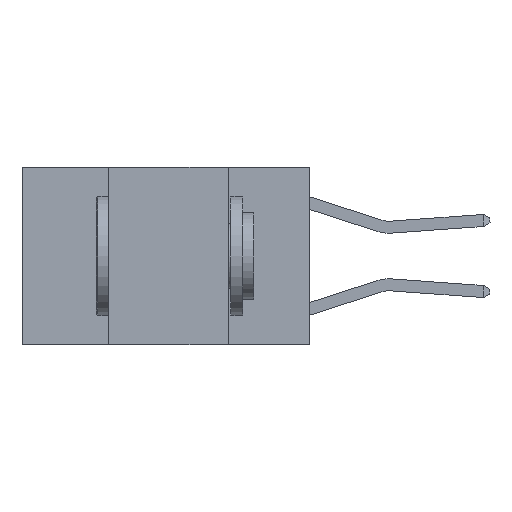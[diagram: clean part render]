
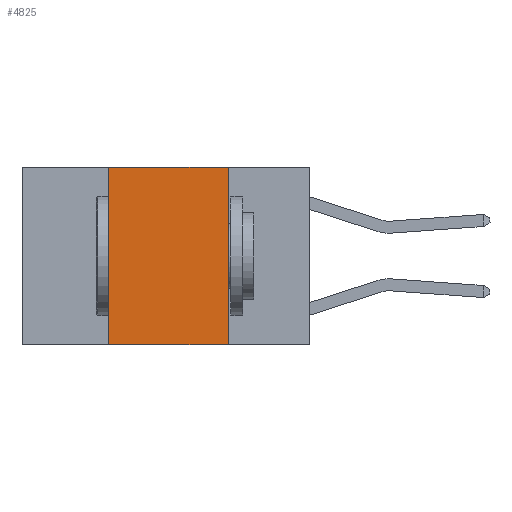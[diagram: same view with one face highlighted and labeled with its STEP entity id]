
A CAD part, left-side view. The second image highlights one B-rep face of the part: STEP entity #4825.
In plain terms, the highlighted planar face has unit normal (-1, 0, 0).
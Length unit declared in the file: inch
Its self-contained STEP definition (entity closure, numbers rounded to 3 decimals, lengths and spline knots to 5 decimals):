
#634 = VECTOR ( 'NONE', #3874, 39.37008 ) ;
#703 = VERTEX_POINT ( 'NONE', #14849 ) ;
#2016 = AXIS2_PLACEMENT_3D ( 'NONE', #13843, #4332, #15391 ) ;
#2614 = DIRECTION ( 'NONE',  ( 0., 0., 1. ) ) ;
#3172 = CARTESIAN_POINT ( 'NONE',  ( 0., 0.42, 0. ) ) ;
#3627 = CARTESIAN_POINT ( 'NONE',  ( 0., 0.6, -0.37 ) ) ;
#3639 = VECTOR ( 'NONE', #2614, 39.37008 ) ;
#3651 = ORIENTED_EDGE ( 'NONE', *, *, #3900, .F. ) ;
#3874 = DIRECTION ( 'NONE',  ( 0., 0., -1. ) ) ;
#3900 = EDGE_CURVE ( 'NONE', #703, #5578, #4510, .T. ) ;
#3946 = ORIENTED_EDGE ( 'NONE', *, *, #17797, .F. ) ;
#4332 = DIRECTION ( 'NONE',  ( 1., 0., 0. ) ) ;
#4471 = ORIENTED_EDGE ( 'NONE', *, *, #7173, .F. ) ;
#4510 = LINE ( 'NONE', #13406, #634 ) ;
#4579 = ORIENTED_EDGE ( 'NONE', *, *, #13881, .T. ) ;
#4668 = CARTESIAN_POINT ( 'NONE',  ( 0., 0.17, -0.37 ) ) ;
#4825 = ADVANCED_FACE ( 'NONE', ( #5985 ), #18412, .F. ) ;
#5578 = VERTEX_POINT ( 'NONE', #4668 ) ;
#5985 = FACE_OUTER_BOUND ( 'NONE', #7747, .T. ) ;
#7173 = EDGE_CURVE ( 'NONE', #14962, #12348, #12115, .T. ) ;
#7747 = EDGE_LOOP ( 'NONE', ( #3651, #3946, #4471, #4579 ) ) ;
#8236 = VECTOR ( 'NONE', #11451, 39.37008 ) ;
#11382 = CARTESIAN_POINT ( 'NONE',  ( 0., 0.6, 0. ) ) ;
#11451 = DIRECTION ( 'NONE',  ( 0., -1., 0. ) ) ;
#12115 = LINE ( 'NONE', #12200, #3639 ) ;
#12200 = CARTESIAN_POINT ( 'NONE',  ( 0., 0.42, 0. ) ) ;
#12348 = VERTEX_POINT ( 'NONE', #3172 ) ;
#12413 = LINE ( 'NONE', #11382, #8236 ) ;
#13406 = CARTESIAN_POINT ( 'NONE',  ( 0., 0.17, 0. ) ) ;
#13843 = CARTESIAN_POINT ( 'NONE',  ( 0., 0.6, 0. ) ) ;
#13881 = EDGE_CURVE ( 'NONE', #14962, #5578, #15448, .T. ) ;
#14715 = DIRECTION ( 'NONE',  ( 0., -1., 0. ) ) ;
#14849 = CARTESIAN_POINT ( 'NONE',  ( 0., 0.17, 0. ) ) ;
#14962 = VERTEX_POINT ( 'NONE', #17401 ) ;
#15391 = DIRECTION ( 'NONE',  ( 0., 0., -1. ) ) ;
#15448 = LINE ( 'NONE', #3627, #19537 ) ;
#17401 = CARTESIAN_POINT ( 'NONE',  ( 0., 0.42, -0.37 ) ) ;
#17797 = EDGE_CURVE ( 'NONE', #12348, #703, #12413, .T. ) ;
#18412 = PLANE ( 'NONE',  #2016 ) ;
#19537 = VECTOR ( 'NONE', #14715, 39.37008 ) ;
